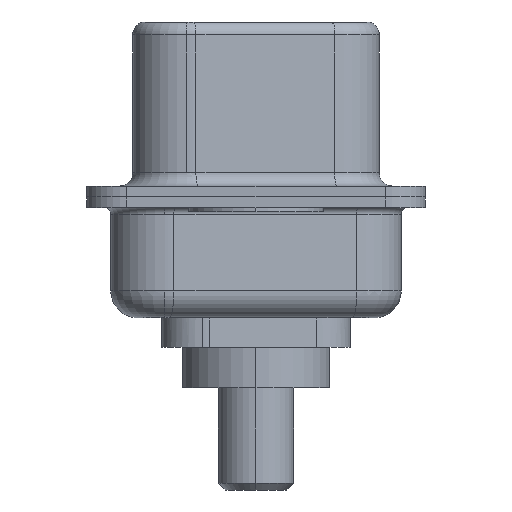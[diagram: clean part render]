
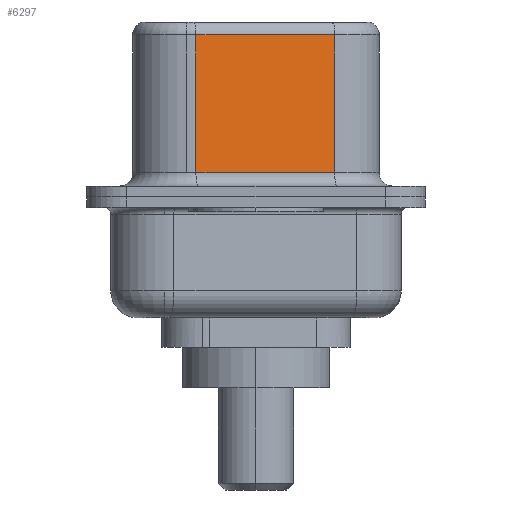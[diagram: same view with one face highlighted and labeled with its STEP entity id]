
A CAD part, left-side view. The second image highlights one B-rep face of the part: STEP entity #6297.
In plain terms, the highlighted planar face has unit normal (-0.985, -0.174, 0).
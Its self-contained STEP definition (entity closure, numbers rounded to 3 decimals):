
#371 = CARTESIAN_POINT ( 'NONE',  ( 4.585, -2.927, 0.9 ) ) ;
#613 = VECTOR ( 'NONE', #2289, 1000. ) ;
#742 = VERTEX_POINT ( 'NONE', #9293 ) ;
#795 = VECTOR ( 'NONE', #2317, 1000. ) ;
#1090 = LINE ( 'NONE', #5524, #6286 ) ;
#1963 = EDGE_LOOP ( 'NONE', ( #4059, #7099, #2171, #5033 ) ) ;
#2171 = ORIENTED_EDGE ( 'NONE', *, *, #11248, .T. ) ;
#2289 = DIRECTION ( 'NONE',  ( -0.174, 0.985, 0. ) ) ;
#2317 = DIRECTION ( 'NONE',  ( 0., 0., -1. ) ) ;
#2378 = DIRECTION ( 'NONE',  ( -0.174, 0.985, 0. ) ) ;
#2684 = FACE_OUTER_BOUND ( 'NONE', #1963, .T. ) ;
#3215 = LINE ( 'NONE', #6013, #613 ) ;
#3325 = VECTOR ( 'NONE', #6252, 1000. ) ;
#3337 = CARTESIAN_POINT ( 'NONE',  ( 3.675, 2.233, 6.52 ) ) ;
#4059 = ORIENTED_EDGE ( 'NONE', *, *, #7203, .F. ) ;
#5033 = ORIENTED_EDGE ( 'NONE', *, *, #7144, .T. ) ;
#5174 = AXIS2_PLACEMENT_3D ( 'NONE', #6023, #8104, #2378 ) ;
#5524 = CARTESIAN_POINT ( 'NONE',  ( 4.585, -2.927, 0.9 ) ) ;
#5828 = CARTESIAN_POINT ( 'NONE',  ( 4.585, -2.927, 6.52 ) ) ;
#6013 = CARTESIAN_POINT ( 'NONE',  ( 4.585, -2.927, 6.02 ) ) ;
#6023 = CARTESIAN_POINT ( 'NONE',  ( 4.585, -2.927, 6.52 ) ) ;
#6252 = DIRECTION ( 'NONE',  ( 0., 0., -1. ) ) ;
#6286 = VECTOR ( 'NONE', #10281, 1000. ) ;
#6297 = ADVANCED_FACE ( 'NONE', ( #2684 ), #11423, .F. ) ;
#6994 = VERTEX_POINT ( 'NONE', #371 ) ;
#7035 = VERTEX_POINT ( 'NONE', #8467 ) ;
#7099 = ORIENTED_EDGE ( 'NONE', *, *, #8603, .T. ) ;
#7144 = EDGE_CURVE ( 'NONE', #9187, #6994, #1090, .T. ) ;
#7203 = EDGE_CURVE ( 'NONE', #742, #6994, #11091, .T. ) ;
#8104 = DIRECTION ( 'NONE',  ( 0.985, 0.174, 0. ) ) ;
#8467 = CARTESIAN_POINT ( 'NONE',  ( 3.675, 2.233, 6.02 ) ) ;
#8603 = EDGE_CURVE ( 'NONE', #742, #7035, #3215, .T. ) ;
#8773 = LINE ( 'NONE', #3337, #3325 ) ;
#9187 = VERTEX_POINT ( 'NONE', #10465 ) ;
#9293 = CARTESIAN_POINT ( 'NONE',  ( 4.585, -2.927, 6.02 ) ) ;
#10281 = DIRECTION ( 'NONE',  ( 0.174, -0.985, 0. ) ) ;
#10465 = CARTESIAN_POINT ( 'NONE',  ( 3.675, 2.233, 0.9 ) ) ;
#11091 = LINE ( 'NONE', #5828, #795 ) ;
#11248 = EDGE_CURVE ( 'NONE', #7035, #9187, #8773, .T. ) ;
#11423 = PLANE ( 'NONE',  #5174 ) ;
